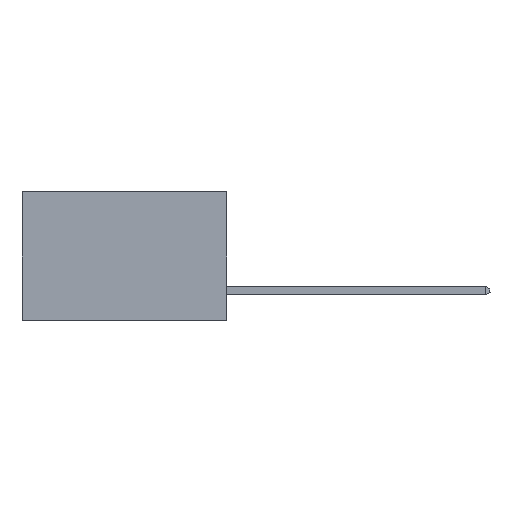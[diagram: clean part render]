
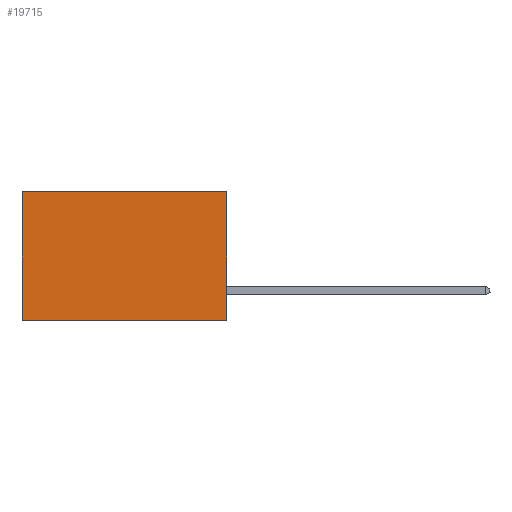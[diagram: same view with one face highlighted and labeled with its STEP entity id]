
A CAD part, left-side view. The second image highlights one B-rep face of the part: STEP entity #19715.
In plain terms, the highlighted planar face has unit normal (-1, 0, 0).
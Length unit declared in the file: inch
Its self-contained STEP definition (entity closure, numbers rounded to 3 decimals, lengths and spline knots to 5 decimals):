
#23 = CARTESIAN_POINT ( 'NONE',  ( 0.277, 0., -0.37 ) ) ;
#32 = LINE ( 'NONE', #23, #19259 ) ;
#444 = ORIENTED_EDGE ( 'NONE', *, *, #11327, .F. ) ;
#606 = CARTESIAN_POINT ( 'NONE',  ( 0.277, 0.59, 0. ) ) ;
#3835 = CARTESIAN_POINT ( 'NONE',  ( 0.277, 0., -0.37 ) ) ;
#4330 = DIRECTION ( 'NONE',  ( 0., 0., -1. ) ) ;
#5333 = LINE ( 'NONE', #7483, #19427 ) ;
#5429 = ORIENTED_EDGE ( 'NONE', *, *, #7557, .F. ) ;
#5592 = VERTEX_POINT ( 'NONE', #606 ) ;
#6867 = FACE_OUTER_BOUND ( 'NONE', #15735, .T. ) ;
#7440 = VECTOR ( 'NONE', #10216, 39.37008 ) ;
#7483 = CARTESIAN_POINT ( 'NONE',  ( 0.277, 0.59, -0.37 ) ) ;
#7557 = EDGE_CURVE ( 'NONE', #10644, #12802, #17592, .T. ) ;
#7565 = DIRECTION ( 'NONE',  ( 0., 0., -1. ) ) ;
#7739 = VECTOR ( 'NONE', #4330, 39.37008 ) ;
#7777 = EDGE_CURVE ( 'NONE', #10644, #5592, #22026, .T. ) ;
#7975 = CARTESIAN_POINT ( 'NONE',  ( 0.277, 0.59, -0.37 ) ) ;
#8022 = CARTESIAN_POINT ( 'NONE',  ( 0.277, 0., -0.37 ) ) ;
#8261 = ORIENTED_EDGE ( 'NONE', *, *, #7777, .T. ) ;
#10216 = DIRECTION ( 'NONE',  ( 0., 1., 0. ) ) ;
#10644 = VERTEX_POINT ( 'NONE', #18078 ) ;
#11131 = CARTESIAN_POINT ( 'NONE',  ( 0.277, 0., 0. ) ) ;
#11327 = EDGE_CURVE ( 'NONE', #12802, #15523, #32, .T. ) ;
#12802 = VERTEX_POINT ( 'NONE', #18238 ) ;
#13158 = DIRECTION ( 'NONE',  ( 0., 1., 0. ) ) ;
#14941 = DIRECTION ( 'NONE',  ( 0., 0., -1. ) ) ;
#15341 = EDGE_CURVE ( 'NONE', #5592, #15523, #5333, .T. ) ;
#15523 = VERTEX_POINT ( 'NONE', #7975 ) ;
#15735 = EDGE_LOOP ( 'NONE', ( #20154, #444, #5429, #8261 ) ) ;
#16731 = PLANE ( 'NONE',  #19772 ) ;
#17592 = LINE ( 'NONE', #8022, #7739 ) ;
#18078 = CARTESIAN_POINT ( 'NONE',  ( 0.277, 0., 0. ) ) ;
#18238 = CARTESIAN_POINT ( 'NONE',  ( 0.277, 0., -0.37 ) ) ;
#18616 = DIRECTION ( 'NONE',  ( 1., 0., 0. ) ) ;
#19259 = VECTOR ( 'NONE', #13158, 39.37008 ) ;
#19427 = VECTOR ( 'NONE', #14941, 39.37008 ) ;
#19715 = ADVANCED_FACE ( 'NONE', ( #6867 ), #16731, .F. ) ;
#19772 = AXIS2_PLACEMENT_3D ( 'NONE', #3835, #18616, #7565 ) ;
#20154 = ORIENTED_EDGE ( 'NONE', *, *, #15341, .T. ) ;
#22026 = LINE ( 'NONE', #11131, #7440 ) ;
